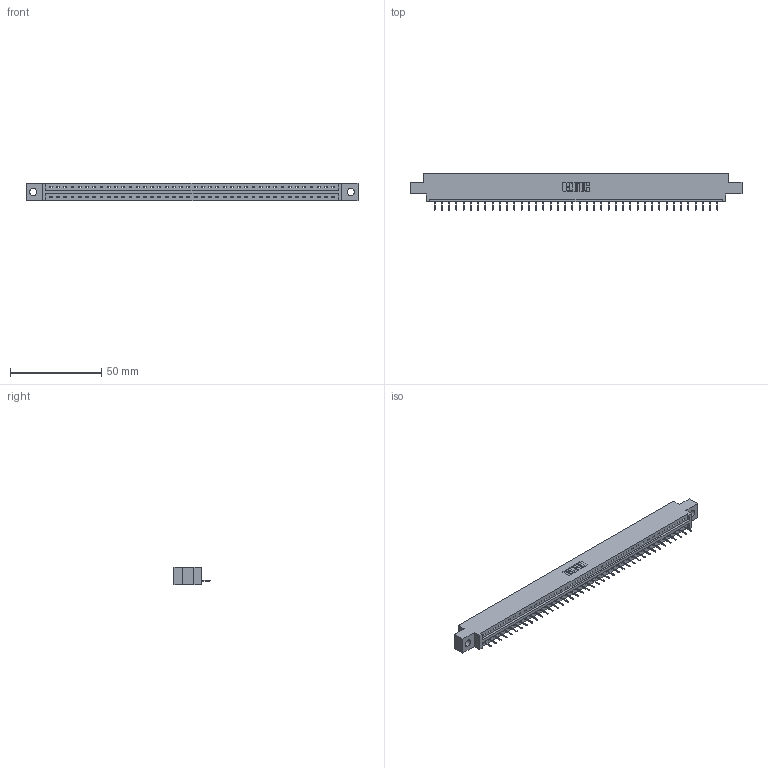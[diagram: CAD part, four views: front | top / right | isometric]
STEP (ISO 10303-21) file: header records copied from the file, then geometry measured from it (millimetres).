
FILE_DESCRIPTION (( 'STEP AP203' ), '1' );
FILE_NAME ('337-040-524-604.STEP', '2018-08-08T10:16:20', ( '' ), ( '' ), 'SwSTEP 2.0', 'SolidWorks 2016', '' );
FILE_SCHEMA (( 'CONFIG_CONTROL_DESIGN' ));
Length unit declared in the file: inch
Products named in the file (3): 337-040-524-604; 337 Part_0.170 Offset - 0.156 Dia-TH; 345-292-001_345-293-124
Assembly tree (41 placements, depth 2):
  337-040-524-604
    337 Part_0.170 Offset - 0.156 Dia-TH
    345-292-001_345-293-124  x40
Bounding box: 181.51 x 19.69 x 9.4 mm (x, y, z)
Volume: 18476.4 mm3; surface area: 18417.5 mm2
Topology: 41 solids, 41 shells, 2758 faces, 8003 edges, 5174 vertices
Faces by surface type: plane 2154, cylinder 604
Entity records: 30201 total; most frequent: CARTESIAN_POINT 5266, ORIENTED_EDGE 5242, DIRECTION 4437, EDGE_CURVE 2621, VECTOR 2497, LINE 2497, VERTEX_POINT 1742, AXIS2_PLACEMENT_3D 970
